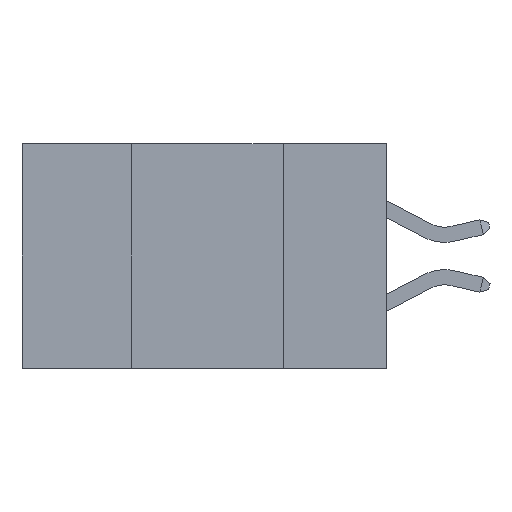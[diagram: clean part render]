
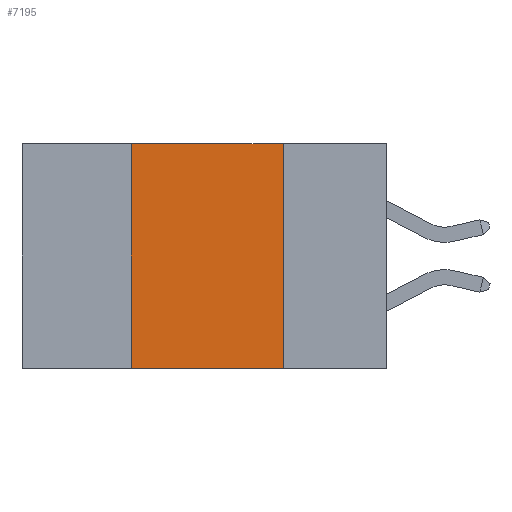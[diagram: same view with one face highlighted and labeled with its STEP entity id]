
A CAD part, left-side view. The second image highlights one B-rep face of the part: STEP entity #7195.
In plain terms, the highlighted planar face has unit normal (-1, 0, 0).
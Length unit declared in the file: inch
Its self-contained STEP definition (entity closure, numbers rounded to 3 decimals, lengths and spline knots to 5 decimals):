
#223 = ORIENTED_EDGE ( 'NONE', *, *, #1759, .T. ) ;
#439 = DIRECTION ( 'NONE',  ( 0., -1., 0. ) ) ;
#1235 = ORIENTED_EDGE ( 'NONE', *, *, #11667, .F. ) ;
#1689 = VECTOR ( 'NONE', #10005, 39.37008 ) ;
#1759 = EDGE_CURVE ( 'NONE', #2563, #13400, #3569, .T. ) ;
#2211 = DIRECTION ( 'NONE',  ( 0., 0., -1. ) ) ;
#2254 = ORIENTED_EDGE ( 'NONE', *, *, #8322, .F. ) ;
#2384 = CARTESIAN_POINT ( 'NONE',  ( 0., 0.17, -0.37 ) ) ;
#2563 = VERTEX_POINT ( 'NONE', #8704 ) ;
#2894 = VECTOR ( 'NONE', #439, 39.37008 ) ;
#3017 = VERTEX_POINT ( 'NONE', #13845 ) ;
#3569 = LINE ( 'NONE', #9380, #1689 ) ;
#4020 = VECTOR ( 'NONE', #7436, 39.37008 ) ;
#4658 = AXIS2_PLACEMENT_3D ( 'NONE', #12128, #5607, #2211 ) ;
#4977 = FACE_OUTER_BOUND ( 'NONE', #12480, .T. ) ;
#5607 = DIRECTION ( 'NONE',  ( 1., 0., 0. ) ) ;
#5854 = CARTESIAN_POINT ( 'NONE',  ( 0., 0.6, 0. ) ) ;
#6434 = LINE ( 'NONE', #7611, #13108 ) ;
#6826 = VERTEX_POINT ( 'NONE', #11065 ) ;
#7195 = ADVANCED_FACE ( 'NONE', ( #4977 ), #12235, .F. ) ;
#7436 = DIRECTION ( 'NONE',  ( 0., 0., -1. ) ) ;
#7611 = CARTESIAN_POINT ( 'NONE',  ( 0., 0.42, 0. ) ) ;
#7836 = ORIENTED_EDGE ( 'NONE', *, *, #10708, .F. ) ;
#8322 = EDGE_CURVE ( 'NONE', #3017, #13400, #9941, .T. ) ;
#8704 = CARTESIAN_POINT ( 'NONE',  ( 0., 0.42, -0.37 ) ) ;
#8804 = LINE ( 'NONE', #5854, #2894 ) ;
#9380 = CARTESIAN_POINT ( 'NONE',  ( 0., 0.6, -0.37 ) ) ;
#9824 = DIRECTION ( 'NONE',  ( 0., 0., 1. ) ) ;
#9941 = LINE ( 'NONE', #13974, #4020 ) ;
#10005 = DIRECTION ( 'NONE',  ( 0., -1., 0. ) ) ;
#10708 = EDGE_CURVE ( 'NONE', #2563, #6826, #6434, .T. ) ;
#11065 = CARTESIAN_POINT ( 'NONE',  ( 0., 0.42, 0. ) ) ;
#11667 = EDGE_CURVE ( 'NONE', #6826, #3017, #8804, .T. ) ;
#12128 = CARTESIAN_POINT ( 'NONE',  ( 0., 0.6, 0. ) ) ;
#12235 = PLANE ( 'NONE',  #4658 ) ;
#12480 = EDGE_LOOP ( 'NONE', ( #2254, #1235, #7836, #223 ) ) ;
#13108 = VECTOR ( 'NONE', #9824, 39.37008 ) ;
#13400 = VERTEX_POINT ( 'NONE', #2384 ) ;
#13845 = CARTESIAN_POINT ( 'NONE',  ( 0., 0.17, 0. ) ) ;
#13974 = CARTESIAN_POINT ( 'NONE',  ( 0., 0.17, 0. ) ) ;
